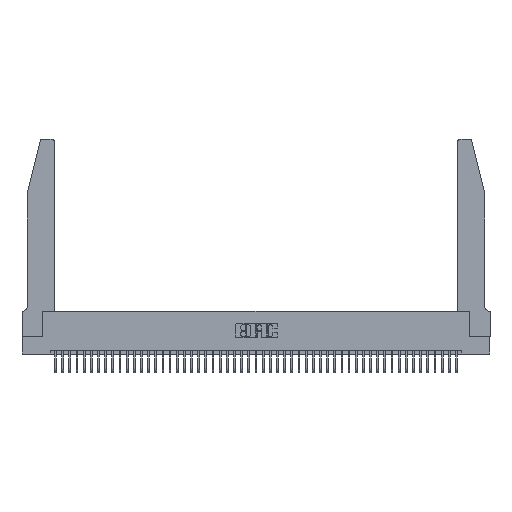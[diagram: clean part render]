
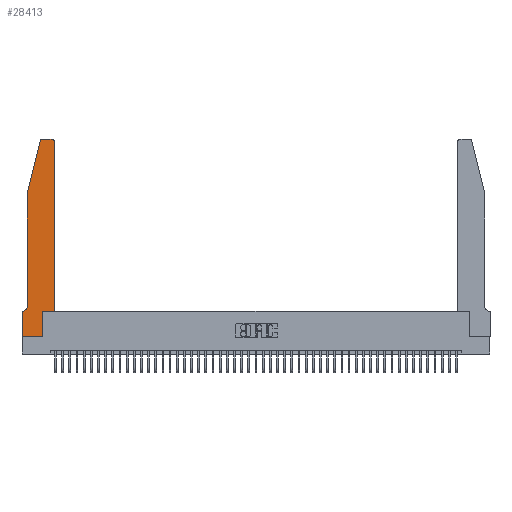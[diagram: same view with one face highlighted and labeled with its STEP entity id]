
A CAD part, top view. The second image highlights one B-rep face of the part: STEP entity #28413.
In plain terms, the highlighted planar face has unit normal (0, 0, 1).
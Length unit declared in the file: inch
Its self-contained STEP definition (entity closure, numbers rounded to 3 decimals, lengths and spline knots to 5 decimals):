
#591 = CARTESIAN_POINT ( 'NONE',  ( 0.0055, 0.42, 0.37 ) ) ;
#984 = DIRECTION ( 'NONE',  ( 1., 0., 0. ) ) ;
#1310 = CIRCLE ( 'NONE', #7102, 0.03 ) ;
#2196 = CARTESIAN_POINT ( 'NONE',  ( 0.2865, 0.35, 0.37 ) ) ;
#2214 = ORIENTED_EDGE ( 'NONE', *, *, #30410, .T. ) ;
#2626 = EDGE_CURVE ( 'NONE', #9480, #27490, #17616, .T. ) ;
#2639 = ORIENTED_EDGE ( 'NONE', *, *, #2626, .T. ) ;
#3001 = EDGE_LOOP ( 'NONE', ( #21212, #41857, #33927, #10805, #26866, #26033, #2639, #2214, #7224, #37059, #22609, #26493 ) ) ;
#3279 = VERTEX_POINT ( 'NONE', #7945 ) ;
#4166 = DIRECTION ( 'NONE',  ( -1., 0., 0. ) ) ;
#6178 = CARTESIAN_POINT ( 'NONE',  ( 0., 0.35, 0.37 ) ) ;
#6351 = DIRECTION ( 'NONE',  ( 1., 0., 0. ) ) ;
#7017 = CARTESIAN_POINT ( 'NONE',  ( 0.0055, 0.35, 0.37 ) ) ;
#7102 = AXIS2_PLACEMENT_3D ( 'NONE', #43266, #22089, #984 ) ;
#7224 = ORIENTED_EDGE ( 'NONE', *, *, #10921, .T. ) ;
#7945 = CARTESIAN_POINT ( 'NONE',  ( 0.4505, 2.72, 0.37 ) ) ;
#8107 = EDGE_CURVE ( 'NONE', #34579, #29501, #38424, .T. ) ;
#8461 = CARTESIAN_POINT ( 'NONE',  ( 0.284, 2.75, 0.37 ) ) ;
#9480 = VERTEX_POINT ( 'NONE', #6178 ) ;
#9594 = EDGE_CURVE ( 'NONE', #35962, #34579, #26068, .T. ) ;
#9732 = CARTESIAN_POINT ( 'NONE',  ( 0., 0., 0.37 ) ) ;
#10118 = LINE ( 'NONE', #9732, #27735 ) ;
#10805 = ORIENTED_EDGE ( 'NONE', *, *, #13910, .T. ) ;
#10921 = EDGE_CURVE ( 'NONE', #27211, #43761, #37113, .T. ) ;
#11084 = CARTESIAN_POINT ( 'NONE',  ( 0.4505, 0.35, 0.37 ) ) ;
#11191 = VECTOR ( 'NONE', #21359, 39.37008 ) ;
#11424 = DIRECTION ( 'NONE',  ( 0., -1., 0. ) ) ;
#12285 = VECTOR ( 'NONE', #18496, 39.37008 ) ;
#13910 = EDGE_CURVE ( 'NONE', #29501, #45205, #37068, .T. ) ;
#14465 = CARTESIAN_POINT ( 'NONE',  ( 0., 0., 0.37 ) ) ;
#14633 = DIRECTION ( 'NONE',  ( 0., 1., 0. ) ) ;
#15022 = LINE ( 'NONE', #27410, #24369 ) ;
#15421 = VERTEX_POINT ( 'NONE', #33973 ) ;
#16099 = CARTESIAN_POINT ( 'NONE',  ( 0.4205, 2.75, 0.37 ) ) ;
#16345 = EDGE_CURVE ( 'NONE', #15421, #3279, #22405, .T. ) ;
#16786 = CARTESIAN_POINT ( 'NONE',  ( 0.2865, 0., 0.37 ) ) ;
#17396 = VECTOR ( 'NONE', #34376, 39.37008 ) ;
#17516 = DIRECTION ( 'NONE',  ( 0., 0., 1. ) ) ;
#17616 = LINE ( 'NONE', #14465, #11191 ) ;
#18249 = CARTESIAN_POINT ( 'NONE',  ( 0.0755, 2., 0.37 ) ) ;
#18496 = DIRECTION ( 'NONE',  ( 0., 1., 0. ) ) ;
#19219 = CARTESIAN_POINT ( 'NONE',  ( 0.25487, 2.72718, 0.37 ) ) ;
#20839 = CARTESIAN_POINT ( 'NONE',  ( 0., 0.35, 0.37 ) ) ;
#21212 = ORIENTED_EDGE ( 'NONE', *, *, #21790, .T. ) ;
#21359 = DIRECTION ( 'NONE',  ( 0., -1., 0. ) ) ;
#21790 = EDGE_CURVE ( 'NONE', #26078, #35962, #27892, .T. ) ;
#22009 = CARTESIAN_POINT ( 'NONE',  ( 0., 0., 0.37 ) ) ;
#22089 = DIRECTION ( 'NONE',  ( 0., 0., 1. ) ) ;
#22405 = LINE ( 'NONE', #11084, #23505 ) ;
#22609 = ORIENTED_EDGE ( 'NONE', *, *, #16345, .T. ) ;
#23505 = VECTOR ( 'NONE', #14633, 39.37008 ) ;
#24369 = VECTOR ( 'NONE', #6351, 39.37008 ) ;
#24384 = PLANE ( 'NONE',  #35218 ) ;
#25238 = DIRECTION ( 'NONE',  ( 0., 0., -1. ) ) ;
#25715 = LINE ( 'NONE', #42504, #44533 ) ;
#26033 = ORIENTED_EDGE ( 'NONE', *, *, #36417, .T. ) ;
#26068 = CIRCLE ( 'NONE', #31638, 0.03 ) ;
#26078 = VERTEX_POINT ( 'NONE', #16099 ) ;
#26493 = ORIENTED_EDGE ( 'NONE', *, *, #39470, .T. ) ;
#26866 = ORIENTED_EDGE ( 'NONE', *, *, #41223, .T. ) ;
#27211 = VERTEX_POINT ( 'NONE', #16786 ) ;
#27410 = CARTESIAN_POINT ( 'NONE',  ( 0.4505, 0.35, 0.37 ) ) ;
#27490 = VERTEX_POINT ( 'NONE', #22009 ) ;
#27735 = VECTOR ( 'NONE', #41509, 39.37008 ) ;
#27792 = CARTESIAN_POINT ( 'NONE',  ( 0.0755, 0.42, 0.37 ) ) ;
#27892 = LINE ( 'NONE', #30791, #17396 ) ;
#27948 = DIRECTION ( 'NONE',  ( 1., 0., 0. ) ) ;
#28413 = ADVANCED_FACE ( 'NONE', ( #37300 ), #24384, .T. ) ;
#29501 = VERTEX_POINT ( 'NONE', #18249 ) ;
#30410 = EDGE_CURVE ( 'NONE', #27490, #27211, #10118, .T. ) ;
#30791 = CARTESIAN_POINT ( 'NONE',  ( 0.2605, 2.75, 0.37 ) ) ;
#31638 = AXIS2_PLACEMENT_3D ( 'NONE', #38723, #17516, #42249 ) ;
#31807 = DIRECTION ( 'NONE',  ( -0.239, -0.971, 0. ) ) ;
#33927 = ORIENTED_EDGE ( 'NONE', *, *, #8107, .T. ) ;
#33973 = CARTESIAN_POINT ( 'NONE',  ( 0.4505, 0.35, 0.37 ) ) ;
#34376 = DIRECTION ( 'NONE',  ( -1., 0., 0. ) ) ;
#34579 = VERTEX_POINT ( 'NONE', #19219 ) ;
#35218 = AXIS2_PLACEMENT_3D ( 'NONE', #20839, #38498, #27948 ) ;
#35375 = CARTESIAN_POINT ( 'NONE',  ( 0.0755, 2., 0.37 ) ) ;
#35417 = DIRECTION ( 'NONE',  ( -1., 0., 0. ) ) ;
#35811 = AXIS2_PLACEMENT_3D ( 'NONE', #591, #25238, #4166 ) ;
#35958 = VECTOR ( 'NONE', #11424, 39.37008 ) ;
#35962 = VERTEX_POINT ( 'NONE', #8461 ) ;
#36417 = EDGE_CURVE ( 'NONE', #36883, #9480, #25715, .T. ) ;
#36883 = VERTEX_POINT ( 'NONE', #7017 ) ;
#37059 = ORIENTED_EDGE ( 'NONE', *, *, #40245, .T. ) ;
#37068 = LINE ( 'NONE', #42573, #35958 ) ;
#37113 = LINE ( 'NONE', #39684, #12285 ) ;
#37300 = FACE_OUTER_BOUND ( 'NONE', #3001, .T. ) ;
#38424 = LINE ( 'NONE', #35375, #45560 ) ;
#38498 = DIRECTION ( 'NONE',  ( 0., 0., 1. ) ) ;
#38723 = CARTESIAN_POINT ( 'NONE',  ( 0.284, 2.72, 0.37 ) ) ;
#39470 = EDGE_CURVE ( 'NONE', #3279, #26078, #1310, .T. ) ;
#39684 = CARTESIAN_POINT ( 'NONE',  ( 0.2865, 0.35, 0.37 ) ) ;
#40245 = EDGE_CURVE ( 'NONE', #43761, #15421, #15022, .T. ) ;
#41223 = EDGE_CURVE ( 'NONE', #45205, #36883, #44733, .T. ) ;
#41509 = DIRECTION ( 'NONE',  ( 1., 0., 0. ) ) ;
#41857 = ORIENTED_EDGE ( 'NONE', *, *, #9594, .T. ) ;
#42249 = DIRECTION ( 'NONE',  ( 1., 0., 0. ) ) ;
#42504 = CARTESIAN_POINT ( 'NONE',  ( 0.0755, 0.35, 0.37 ) ) ;
#42573 = CARTESIAN_POINT ( 'NONE',  ( 0.0755, 2., 0.37 ) ) ;
#43266 = CARTESIAN_POINT ( 'NONE',  ( 0.4205, 2.72, 0.37 ) ) ;
#43761 = VERTEX_POINT ( 'NONE', #2196 ) ;
#44533 = VECTOR ( 'NONE', #35417, 39.37008 ) ;
#44733 = CIRCLE ( 'NONE', #35811, 0.07 ) ;
#45205 = VERTEX_POINT ( 'NONE', #27792 ) ;
#45560 = VECTOR ( 'NONE', #31807, 39.37008 ) ;
